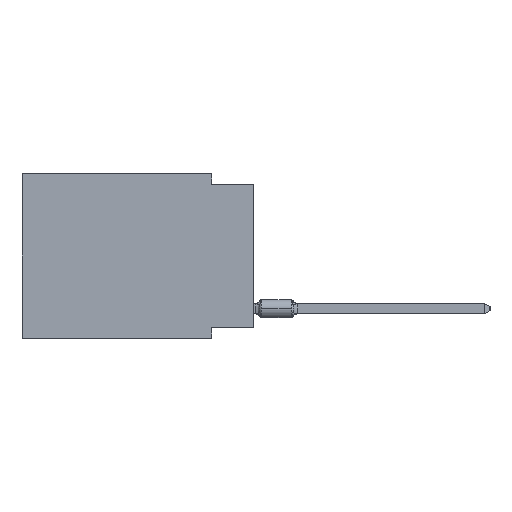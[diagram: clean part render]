
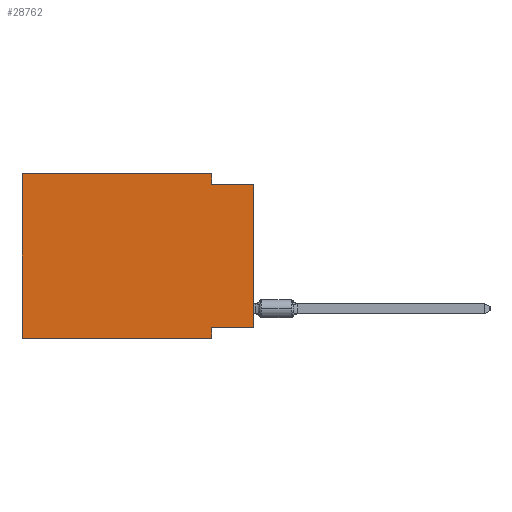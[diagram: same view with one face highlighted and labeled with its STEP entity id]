
A CAD part, left-side view. The second image highlights one B-rep face of the part: STEP entity #28762.
In plain terms, the highlighted planar face has unit normal (-1, 0, 0).
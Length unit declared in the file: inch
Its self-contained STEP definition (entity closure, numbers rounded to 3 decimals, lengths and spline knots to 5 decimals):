
#280 = CARTESIAN_POINT ( 'NONE',  ( 0., 0., 0. ) ) ;
#649 = DIRECTION ( 'NONE',  ( 0., -1., 0. ) ) ;
#1885 = VERTEX_POINT ( 'NONE', #43312 ) ;
#1893 = AXIS2_PLACEMENT_3D ( 'NONE', #3296, #7047, #19654 ) ;
#2733 = ORIENTED_EDGE ( 'NONE', *, *, #48323, .F. ) ;
#3291 = ORIENTED_EDGE ( 'NONE', *, *, #19813, .T. ) ;
#3296 = CARTESIAN_POINT ( 'NONE',  ( 0., 0.55, 0. ) ) ;
#5223 = LINE ( 'NONE', #22989, #34411 ) ;
#5330 = CARTESIAN_POINT ( 'NONE',  ( 0., 0.55, 0. ) ) ;
#6284 = CARTESIAN_POINT ( 'NONE',  ( 0., 0.55, 0. ) ) ;
#6491 = PLANE ( 'NONE',  #1893 ) ;
#7047 = DIRECTION ( 'NONE',  ( 1., 0., 0. ) ) ;
#7081 = VECTOR ( 'NONE', #33328, 39.37008 ) ;
#8644 = CARTESIAN_POINT ( 'NONE',  ( 0., 0., -0.025 ) ) ;
#9219 = VERTEX_POINT ( 'NONE', #21553 ) ;
#9699 = LINE ( 'NONE', #280, #12729 ) ;
#9999 = DIRECTION ( 'NONE',  ( 0., 0., 1. ) ) ;
#10489 = DIRECTION ( 'NONE',  ( 0., 0., 1. ) ) ;
#10496 = EDGE_CURVE ( 'NONE', #1885, #12045, #5223, .T. ) ;
#10808 = VECTOR ( 'NONE', #15587, 39.37008 ) ;
#12045 = VERTEX_POINT ( 'NONE', #8644 ) ;
#12547 = VERTEX_POINT ( 'NONE', #43528 ) ;
#12729 = VECTOR ( 'NONE', #9999, 39.37008 ) ;
#13062 = DIRECTION ( 'NONE',  ( 0., 1., 0. ) ) ;
#13331 = EDGE_LOOP ( 'NONE', ( #3291, #13968, #2733, #15551, #52469, #54204, #32980, #25892 ) ) ;
#13618 = LINE ( 'NONE', #26497, #52181 ) ;
#13968 = ORIENTED_EDGE ( 'NONE', *, *, #10496, .F. ) ;
#14364 = VECTOR ( 'NONE', #10489, 39.37008 ) ;
#15297 = CARTESIAN_POINT ( 'NONE',  ( 0., 0.1, -0.39 ) ) ;
#15551 = ORIENTED_EDGE ( 'NONE', *, *, #51109, .F. ) ;
#15587 = DIRECTION ( 'NONE',  ( 0., 0., -1. ) ) ;
#17865 = EDGE_CURVE ( 'NONE', #23419, #33225, #32759, .T. ) ;
#19321 = DIRECTION ( 'NONE',  ( 0., 0., -1. ) ) ;
#19592 = CARTESIAN_POINT ( 'NONE',  ( 0., 0.55, -0.39 ) ) ;
#19654 = DIRECTION ( 'NONE',  ( 0., 0., -1. ) ) ;
#19813 = EDGE_CURVE ( 'NONE', #51343, #12045, #9699, .T. ) ;
#21553 = CARTESIAN_POINT ( 'NONE',  ( 0., 0.55, 0. ) ) ;
#22989 = CARTESIAN_POINT ( 'NONE',  ( 0., 0., -0.025 ) ) ;
#23419 = VERTEX_POINT ( 'NONE', #54711 ) ;
#25892 = ORIENTED_EDGE ( 'NONE', *, *, #30906, .F. ) ;
#26497 = CARTESIAN_POINT ( 'NONE',  ( 0., 0., -0.365 ) ) ;
#28138 = VECTOR ( 'NONE', #19321, 39.37008 ) ;
#28762 = ADVANCED_FACE ( 'NONE', ( #37411 ), #6491, .F. ) ;
#30906 = EDGE_CURVE ( 'NONE', #51343, #23419, #13618, .T. ) ;
#32759 = LINE ( 'NONE', #15297, #28138 ) ;
#32980 = ORIENTED_EDGE ( 'NONE', *, *, #17865, .F. ) ;
#33225 = VERTEX_POINT ( 'NONE', #55534 ) ;
#33328 = DIRECTION ( 'NONE',  ( 0., -1., 0. ) ) ;
#34411 = VECTOR ( 'NONE', #649, 39.37008 ) ;
#35688 = VECTOR ( 'NONE', #36355, 39.37008 ) ;
#36355 = DIRECTION ( 'NONE',  ( 0., -1., 0. ) ) ;
#37345 = LINE ( 'NONE', #54817, #10808 ) ;
#37411 = FACE_OUTER_BOUND ( 'NONE', #13331, .T. ) ;
#41393 = LINE ( 'NONE', #19592, #7081 ) ;
#41484 = EDGE_CURVE ( 'NONE', #12547, #9219, #49753, .T. ) ;
#43312 = CARTESIAN_POINT ( 'NONE',  ( 0., 0.1, -0.025 ) ) ;
#43528 = CARTESIAN_POINT ( 'NONE',  ( 0., 0.55, -0.39 ) ) ;
#44051 = CARTESIAN_POINT ( 'NONE',  ( 0., 0., -0.365 ) ) ;
#45530 = LINE ( 'NONE', #6284, #35688 ) ;
#48270 = EDGE_CURVE ( 'NONE', #12547, #33225, #41393, .T. ) ;
#48323 = EDGE_CURVE ( 'NONE', #55421, #1885, #37345, .T. ) ;
#49753 = LINE ( 'NONE', #5330, #14364 ) ;
#51109 = EDGE_CURVE ( 'NONE', #9219, #55421, #45530, .T. ) ;
#51343 = VERTEX_POINT ( 'NONE', #44051 ) ;
#52181 = VECTOR ( 'NONE', #13062, 39.37008 ) ;
#52469 = ORIENTED_EDGE ( 'NONE', *, *, #41484, .F. ) ;
#54204 = ORIENTED_EDGE ( 'NONE', *, *, #48270, .T. ) ;
#54711 = CARTESIAN_POINT ( 'NONE',  ( 0., 0.1, -0.365 ) ) ;
#54817 = CARTESIAN_POINT ( 'NONE',  ( 0., 0.1, 0. ) ) ;
#55421 = VERTEX_POINT ( 'NONE', #55956 ) ;
#55534 = CARTESIAN_POINT ( 'NONE',  ( 0., 0.1, -0.39 ) ) ;
#55956 = CARTESIAN_POINT ( 'NONE',  ( 0., 0.1, 0. ) ) ;
